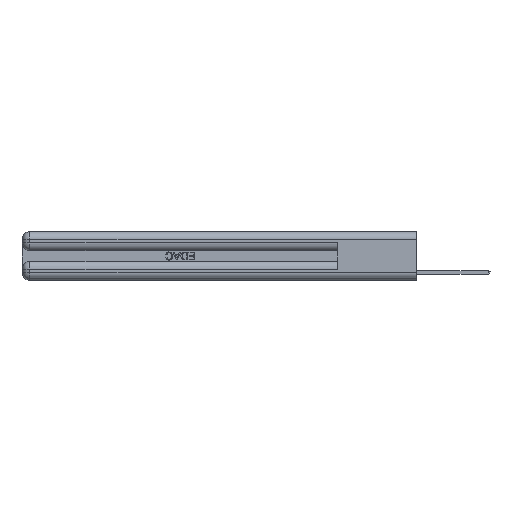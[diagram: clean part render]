
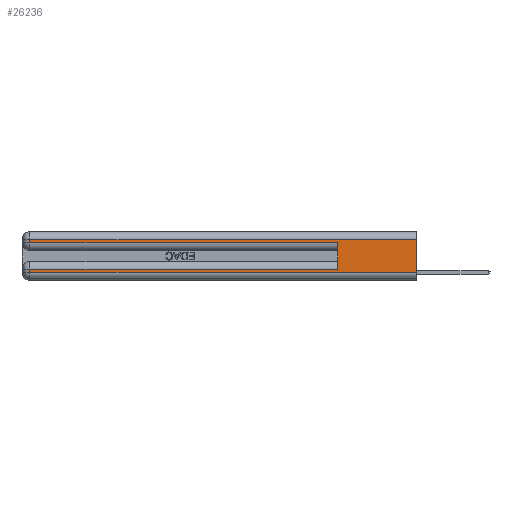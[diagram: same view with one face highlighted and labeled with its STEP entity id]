
A CAD part, left-side view. The second image highlights one B-rep face of the part: STEP entity #26236.
In plain terms, the highlighted planar face has unit normal (-1, 0, 0).
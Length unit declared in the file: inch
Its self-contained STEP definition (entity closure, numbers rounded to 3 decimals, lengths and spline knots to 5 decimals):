
#7 = CARTESIAN_POINT ( 'NONE',  ( 0., 0.6, 0.085 ) ) ;
#626 = LINE ( 'NONE', #5862, #20290 ) ;
#719 = DIRECTION ( 'NONE',  ( 0., -1., 0. ) ) ;
#756 = VERTEX_POINT ( 'NONE', #1746 ) ;
#814 = LINE ( 'NONE', #17930, #6794 ) ;
#852 = EDGE_CURVE ( 'NONE', #1583, #20412, #26592, .T. ) ;
#1583 = VERTEX_POINT ( 'NONE', #7 ) ;
#1611 = LINE ( 'NONE', #21989, #24452 ) ;
#1665 = VERTEX_POINT ( 'NONE', #3254 ) ;
#1746 = CARTESIAN_POINT ( 'NONE',  ( 0., 2.94, 0.31 ) ) ;
#2474 = EDGE_CURVE ( 'NONE', #28392, #23356, #32885, .T. ) ;
#2875 = ORIENTED_EDGE ( 'NONE', *, *, #852, .T. ) ;
#3254 = CARTESIAN_POINT ( 'NONE',  ( 0., 2.94, 0.06 ) ) ;
#3480 = CARTESIAN_POINT ( 'NONE',  ( 0., 0.6, 0.285 ) ) ;
#3759 = EDGE_CURVE ( 'NONE', #1665, #23356, #8717, .T. ) ;
#3894 = VERTEX_POINT ( 'NONE', #3480 ) ;
#4039 = ORIENTED_EDGE ( 'NONE', *, *, #2474, .F. ) ;
#4053 = DIRECTION ( 'NONE',  ( 0., 1., 0. ) ) ;
#5115 = LINE ( 'NONE', #31371, #24367 ) ;
#5639 = CARTESIAN_POINT ( 'NONE',  ( 0., 0., 0.06 ) ) ;
#5862 = CARTESIAN_POINT ( 'NONE',  ( 0., 0., 0.285 ) ) ;
#6794 = VECTOR ( 'NONE', #27844, 39.37008 ) ;
#6806 = ORIENTED_EDGE ( 'NONE', *, *, #25700, .F. ) ;
#7019 = DIRECTION ( 'NONE',  ( 0., 0., -1. ) ) ;
#8717 = LINE ( 'NONE', #5639, #32823 ) ;
#9858 = ORIENTED_EDGE ( 'NONE', *, *, #25398, .T. ) ;
#10135 = CARTESIAN_POINT ( 'NONE',  ( 0., 0., 0.31 ) ) ;
#10679 = EDGE_CURVE ( 'NONE', #756, #18139, #5115, .T. ) ;
#11618 = DIRECTION ( 'NONE',  ( 0., 0., -1. ) ) ;
#13539 = EDGE_LOOP ( 'NONE', ( #4039, #19783, #19288, #28886, #6806, #2875, #9858, #25305 ) ) ;
#13921 = DIRECTION ( 'NONE',  ( 0., 0., -1. ) ) ;
#14978 = PLANE ( 'NONE',  #17200 ) ;
#16937 = VECTOR ( 'NONE', #25423, 39.37008 ) ;
#17200 = AXIS2_PLACEMENT_3D ( 'NONE', #22512, #19823, #7019 ) ;
#17347 = CARTESIAN_POINT ( 'NONE',  ( 0., 2.94, 0.085 ) ) ;
#17930 = CARTESIAN_POINT ( 'NONE',  ( 0., 0.6, 0.145 ) ) ;
#18139 = VERTEX_POINT ( 'NONE', #18364 ) ;
#18364 = CARTESIAN_POINT ( 'NONE',  ( 0., 2.94, 0.285 ) ) ;
#19288 = ORIENTED_EDGE ( 'NONE', *, *, #10679, .T. ) ;
#19783 = ORIENTED_EDGE ( 'NONE', *, *, #29827, .T. ) ;
#19814 = FACE_OUTER_BOUND ( 'NONE', #13539, .T. ) ;
#19823 = DIRECTION ( 'NONE',  ( 1., 0., 0. ) ) ;
#20290 = VECTOR ( 'NONE', #719, 39.37008 ) ;
#20412 = VERTEX_POINT ( 'NONE', #17347 ) ;
#21989 = CARTESIAN_POINT ( 'NONE',  ( 0., 2.94, 0.37 ) ) ;
#22486 = VECTOR ( 'NONE', #11618, 39.37008 ) ;
#22512 = CARTESIAN_POINT ( 'NONE',  ( 0., 0., 0.37 ) ) ;
#23356 = VERTEX_POINT ( 'NONE', #24283 ) ;
#23622 = DIRECTION ( 'NONE',  ( 0., 0., -1. ) ) ;
#24283 = CARTESIAN_POINT ( 'NONE',  ( 0., 0., 0.06 ) ) ;
#24367 = VECTOR ( 'NONE', #23622, 39.37008 ) ;
#24452 = VECTOR ( 'NONE', #13921, 39.37008 ) ;
#25305 = ORIENTED_EDGE ( 'NONE', *, *, #3759, .T. ) ;
#25398 = EDGE_CURVE ( 'NONE', #20412, #1665, #1611, .T. ) ;
#25423 = DIRECTION ( 'NONE',  ( 0., 1., 0. ) ) ;
#25700 = EDGE_CURVE ( 'NONE', #1583, #3894, #814, .T. ) ;
#26236 = ADVANCED_FACE ( 'NONE', ( #19814 ), #14978, .F. ) ;
#26592 = LINE ( 'NONE', #30709, #16937 ) ;
#26830 = CARTESIAN_POINT ( 'NONE',  ( 0., 0., 0.31 ) ) ;
#27457 = EDGE_CURVE ( 'NONE', #18139, #3894, #626, .T. ) ;
#27844 = DIRECTION ( 'NONE',  ( 0., 0., 1. ) ) ;
#28392 = VERTEX_POINT ( 'NONE', #10135 ) ;
#28868 = DIRECTION ( 'NONE',  ( 0., -1., 0. ) ) ;
#28886 = ORIENTED_EDGE ( 'NONE', *, *, #27457, .T. ) ;
#29327 = VECTOR ( 'NONE', #4053, 39.37008 ) ;
#29827 = EDGE_CURVE ( 'NONE', #28392, #756, #31740, .T. ) ;
#30709 = CARTESIAN_POINT ( 'NONE',  ( 0., 0., 0.085 ) ) ;
#31371 = CARTESIAN_POINT ( 'NONE',  ( 0., 2.94, 0.37 ) ) ;
#31510 = CARTESIAN_POINT ( 'NONE',  ( 0., 0., 0.37 ) ) ;
#31740 = LINE ( 'NONE', #26830, #29327 ) ;
#32823 = VECTOR ( 'NONE', #28868, 39.37008 ) ;
#32885 = LINE ( 'NONE', #31510, #22486 ) ;
